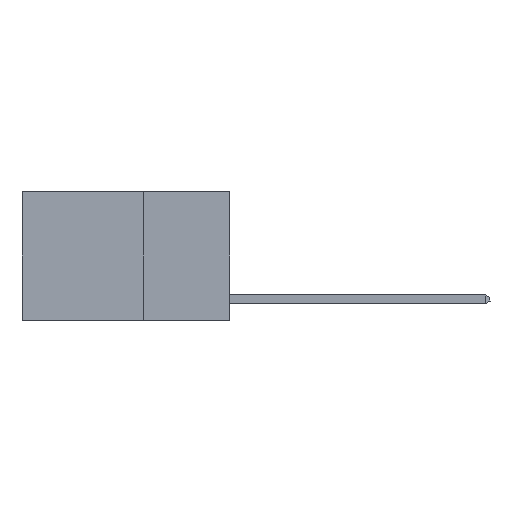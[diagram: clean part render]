
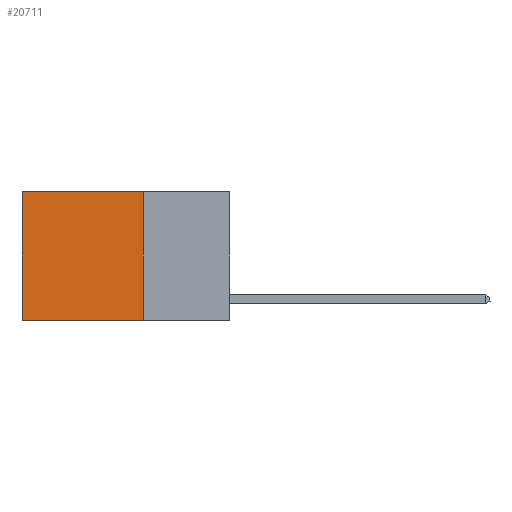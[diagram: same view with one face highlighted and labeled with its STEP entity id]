
A CAD part, left-side view. The second image highlights one B-rep face of the part: STEP entity #20711.
In plain terms, the highlighted planar face has unit normal (-1, 0, 0).
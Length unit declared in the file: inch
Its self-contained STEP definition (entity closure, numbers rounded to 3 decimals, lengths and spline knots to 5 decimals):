
#93 = VERTEX_POINT ( 'NONE', #10014 ) ;
#749 = ORIENTED_EDGE ( 'NONE', *, *, #23466, .F. ) ;
#967 = CARTESIAN_POINT ( 'NONE',  ( 0.2625, 0.6, 0. ) ) ;
#1811 = EDGE_CURVE ( 'NONE', #19922, #8304, #9580, .T. ) ;
#2116 = CARTESIAN_POINT ( 'NONE',  ( 0.2625, 0.25, -0.37 ) ) ;
#2425 = LINE ( 'NONE', #6136, #25169 ) ;
#3465 = DIRECTION ( 'NONE',  ( 0., 0., -1. ) ) ;
#3653 = CARTESIAN_POINT ( 'NONE',  ( 0.2625, 0.25, 0. ) ) ;
#4222 = DIRECTION ( 'NONE',  ( 0., 1., 0. ) ) ;
#4285 = CARTESIAN_POINT ( 'NONE',  ( 0.2625, 0.6, 0. ) ) ;
#4605 = AXIS2_PLACEMENT_3D ( 'NONE', #14950, #4803, #20879 ) ;
#4803 = DIRECTION ( 'NONE',  ( 1., 0., 0. ) ) ;
#5116 = EDGE_CURVE ( 'NONE', #22669, #93, #9262, .T. ) ;
#6136 = CARTESIAN_POINT ( 'NONE',  ( 0.2625, 0.25, 0. ) ) ;
#6387 = VECTOR ( 'NONE', #24783, 39.37008 ) ;
#8304 = VERTEX_POINT ( 'NONE', #9086 ) ;
#9086 = CARTESIAN_POINT ( 'NONE',  ( 0.2625, 0.25, -0.37 ) ) ;
#9262 = LINE ( 'NONE', #967, #19027 ) ;
#9580 = LINE ( 'NONE', #3653, #6387 ) ;
#10014 = CARTESIAN_POINT ( 'NONE',  ( 0.2625, 0.6, -0.37 ) ) ;
#10162 = LINE ( 'NONE', #2116, #21256 ) ;
#10334 = DIRECTION ( 'NONE',  ( 0., 1., 0. ) ) ;
#12154 = ORIENTED_EDGE ( 'NONE', *, *, #19250, .T. ) ;
#12712 = FACE_OUTER_BOUND ( 'NONE', #23579, .T. ) ;
#14950 = CARTESIAN_POINT ( 'NONE',  ( 0.2625, 0.25, 0. ) ) ;
#18265 = ORIENTED_EDGE ( 'NONE', *, *, #1811, .F. ) ;
#18632 = PLANE ( 'NONE',  #4605 ) ;
#19027 = VECTOR ( 'NONE', #3465, 39.37008 ) ;
#19250 = EDGE_CURVE ( 'NONE', #19922, #22669, #2425, .T. ) ;
#19656 = CARTESIAN_POINT ( 'NONE',  ( 0.2625, 0.25, 0. ) ) ;
#19922 = VERTEX_POINT ( 'NONE', #19656 ) ;
#20711 = ADVANCED_FACE ( 'NONE', ( #12712 ), #18632, .F. ) ;
#20879 = DIRECTION ( 'NONE',  ( 0., 0., -1. ) ) ;
#21256 = VECTOR ( 'NONE', #4222, 39.37008 ) ;
#22471 = ORIENTED_EDGE ( 'NONE', *, *, #5116, .T. ) ;
#22669 = VERTEX_POINT ( 'NONE', #4285 ) ;
#23466 = EDGE_CURVE ( 'NONE', #8304, #93, #10162, .T. ) ;
#23579 = EDGE_LOOP ( 'NONE', ( #22471, #749, #18265, #12154 ) ) ;
#24783 = DIRECTION ( 'NONE',  ( 0., 0., -1. ) ) ;
#25169 = VECTOR ( 'NONE', #10334, 39.37008 ) ;
